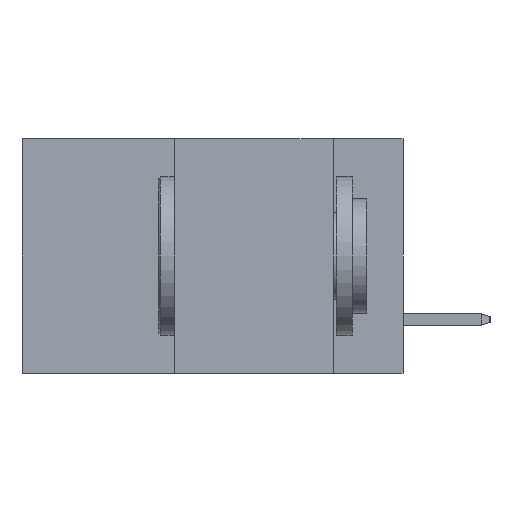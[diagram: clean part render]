
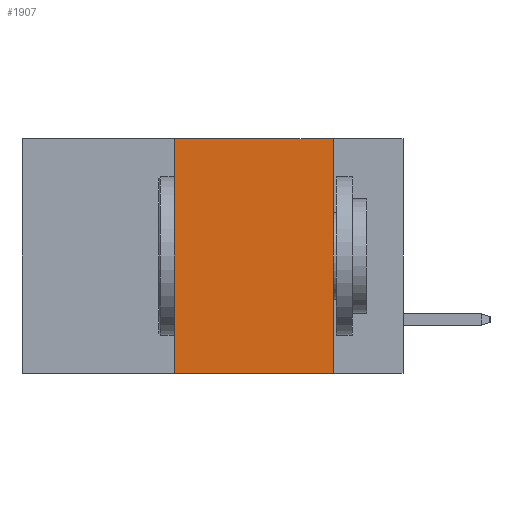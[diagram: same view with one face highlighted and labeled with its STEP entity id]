
A CAD part, left-side view. The second image highlights one B-rep face of the part: STEP entity #1907.
In plain terms, the highlighted planar face has unit normal (-1, 0, 0).
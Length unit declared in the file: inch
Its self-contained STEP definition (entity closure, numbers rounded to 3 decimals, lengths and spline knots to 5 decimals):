
#669 = CARTESIAN_POINT ( 'NONE',  ( 0., 0.6, 0. ) ) ;
#949 = CARTESIAN_POINT ( 'NONE',  ( 0., 0.6, -0.37 ) ) ;
#1283 = VERTEX_POINT ( 'NONE', #12818 ) ;
#1818 = ORIENTED_EDGE ( 'NONE', *, *, #6960, .F. ) ;
#1907 = ADVANCED_FACE ( 'NONE', ( #7552 ), #6570, .F. ) ;
#2289 = EDGE_CURVE ( 'NONE', #3868, #1283, #13406, .T. ) ;
#2353 = VECTOR ( 'NONE', #13843, 39.37008 ) ;
#2681 = CARTESIAN_POINT ( 'NONE',  ( 0., 0.36, -0.37 ) ) ;
#2972 = VERTEX_POINT ( 'NONE', #12519 ) ;
#3302 = VECTOR ( 'NONE', #15804, 39.37008 ) ;
#3868 = VERTEX_POINT ( 'NONE', #11828 ) ;
#5386 = CARTESIAN_POINT ( 'NONE',  ( 0., 0.36, 0. ) ) ;
#5465 = DIRECTION ( 'NONE',  ( 0., 0., 1. ) ) ;
#6570 = PLANE ( 'NONE',  #14501 ) ;
#6960 = EDGE_CURVE ( 'NONE', #9776, #3868, #8865, .T. ) ;
#7505 = EDGE_LOOP ( 'NONE', ( #13357, #12999, #1818, #11914 ) ) ;
#7552 = FACE_OUTER_BOUND ( 'NONE', #7505, .T. ) ;
#8865 = LINE ( 'NONE', #5386, #10763 ) ;
#9013 = CARTESIAN_POINT ( 'NONE',  ( 0., 0.11, 0. ) ) ;
#9429 = LINE ( 'NONE', #949, #15692 ) ;
#9776 = VERTEX_POINT ( 'NONE', #2681 ) ;
#9912 = CARTESIAN_POINT ( 'NONE',  ( 0., 0.6, 0. ) ) ;
#10469 = DIRECTION ( 'NONE',  ( 0., -1., 0. ) ) ;
#10582 = DIRECTION ( 'NONE',  ( 0., 0., -1. ) ) ;
#10763 = VECTOR ( 'NONE', #5465, 39.37008 ) ;
#11324 = EDGE_CURVE ( 'NONE', #1283, #2972, #15148, .T. ) ;
#11828 = CARTESIAN_POINT ( 'NONE',  ( 0., 0.36, 0. ) ) ;
#11914 = ORIENTED_EDGE ( 'NONE', *, *, #13651, .T. ) ;
#12519 = CARTESIAN_POINT ( 'NONE',  ( 0., 0.11, -0.37 ) ) ;
#12818 = CARTESIAN_POINT ( 'NONE',  ( 0., 0.11, 0. ) ) ;
#12999 = ORIENTED_EDGE ( 'NONE', *, *, #2289, .F. ) ;
#13357 = ORIENTED_EDGE ( 'NONE', *, *, #11324, .F. ) ;
#13406 = LINE ( 'NONE', #9912, #3302 ) ;
#13651 = EDGE_CURVE ( 'NONE', #9776, #2972, #9429, .T. ) ;
#13843 = DIRECTION ( 'NONE',  ( 0., 0., -1. ) ) ;
#14501 = AXIS2_PLACEMENT_3D ( 'NONE', #669, #15378, #10582 ) ;
#15148 = LINE ( 'NONE', #9013, #2353 ) ;
#15378 = DIRECTION ( 'NONE',  ( 1., 0., 0. ) ) ;
#15692 = VECTOR ( 'NONE', #10469, 39.37008 ) ;
#15804 = DIRECTION ( 'NONE',  ( 0., -1., 0. ) ) ;
